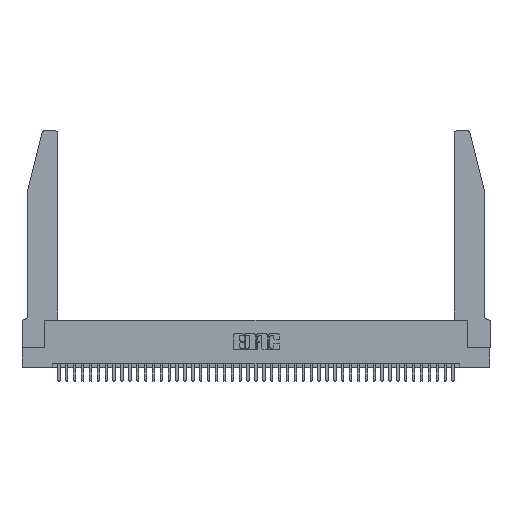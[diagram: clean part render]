
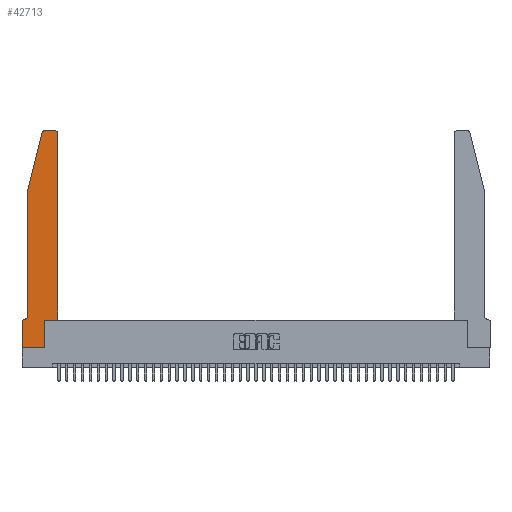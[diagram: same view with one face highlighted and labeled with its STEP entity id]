
A CAD part, top view. The second image highlights one B-rep face of the part: STEP entity #42713.
In plain terms, the highlighted planar face has unit normal (0, 0, 1).
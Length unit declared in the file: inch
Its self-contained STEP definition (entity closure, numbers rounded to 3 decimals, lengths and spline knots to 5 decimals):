
#210 = EDGE_CURVE ( 'NONE', #33803, #3061, #4650, .T. ) ;
#234 = VECTOR ( 'NONE', #22445, 39.37008 ) ;
#853 = DIRECTION ( 'NONE',  ( 1., 0., 0. ) ) ;
#1028 = EDGE_CURVE ( 'NONE', #3170, #3610, #22597, .T. ) ;
#1402 = ORIENTED_EDGE ( 'NONE', *, *, #32171, .T. ) ;
#1412 = VERTEX_POINT ( 'NONE', #35354 ) ;
#1661 = DIRECTION ( 'NONE',  ( 1., 0., 0. ) ) ;
#1755 = ORIENTED_EDGE ( 'NONE', *, *, #35475, .T. ) ;
#2076 = CARTESIAN_POINT ( 'NONE',  ( 0.4505, 0.35, 0.37 ) ) ;
#2695 = LINE ( 'NONE', #10277, #16411 ) ;
#3061 = VERTEX_POINT ( 'NONE', #4089 ) ;
#3170 = VERTEX_POINT ( 'NONE', #8322 ) ;
#3610 = VERTEX_POINT ( 'NONE', #16871 ) ;
#3651 = CARTESIAN_POINT ( 'NONE',  ( 0.284, 2.72, 0.37 ) ) ;
#4089 = CARTESIAN_POINT ( 'NONE',  ( 0.4505, 0.35, 0.37 ) ) ;
#4650 = LINE ( 'NONE', #28960, #7803 ) ;
#5351 = DIRECTION ( 'NONE',  ( -1., 0., 0. ) ) ;
#5510 = DIRECTION ( 'NONE',  ( -0.239, -0.971, 0. ) ) ;
#5765 = VECTOR ( 'NONE', #33285, 39.37008 ) ;
#6436 = DIRECTION ( 'NONE',  ( 0., -1., 0. ) ) ;
#6852 = ORIENTED_EDGE ( 'NONE', *, *, #40280, .T. ) ;
#7072 = AXIS2_PLACEMENT_3D ( 'NONE', #19152, #12638, #22562 ) ;
#7702 = ORIENTED_EDGE ( 'NONE', *, *, #210, .T. ) ;
#7803 = VECTOR ( 'NONE', #1661, 39.37008 ) ;
#8322 = CARTESIAN_POINT ( 'NONE',  ( 0.0755, 2., 0.37 ) ) ;
#8665 = ORIENTED_EDGE ( 'NONE', *, *, #29667, .T. ) ;
#9045 = CARTESIAN_POINT ( 'NONE',  ( 0.2865, 0.35, 0.37 ) ) ;
#9148 = DIRECTION ( 'NONE',  ( 0., 0., 1. ) ) ;
#9233 = CIRCLE ( 'NONE', #14042, 0.03 ) ;
#10057 = ORIENTED_EDGE ( 'NONE', *, *, #18216, .T. ) ;
#10277 = CARTESIAN_POINT ( 'NONE',  ( 0., 0., 0.37 ) ) ;
#11671 = CARTESIAN_POINT ( 'NONE',  ( 0.0755, 2., 0.37 ) ) ;
#12036 = EDGE_CURVE ( 'NONE', #3610, #27990, #17361, .T. ) ;
#12462 = VECTOR ( 'NONE', #39123, 39.37008 ) ;
#12638 = DIRECTION ( 'NONE',  ( 0., 0., 1. ) ) ;
#13542 = EDGE_CURVE ( 'NONE', #27990, #29361, #26884, .T. ) ;
#13628 = CARTESIAN_POINT ( 'NONE',  ( 0., 0.35, 0.37 ) ) ;
#13631 = CARTESIAN_POINT ( 'NONE',  ( 0.2605, 2.75, 0.37 ) ) ;
#14042 = AXIS2_PLACEMENT_3D ( 'NONE', #3651, #20443, #853 ) ;
#14586 = LINE ( 'NONE', #27239, #39975 ) ;
#16258 = AXIS2_PLACEMENT_3D ( 'NONE', #22179, #18629, #5351 ) ;
#16411 = VECTOR ( 'NONE', #20325, 39.37008 ) ;
#16871 = CARTESIAN_POINT ( 'NONE',  ( 0.0755, 0.42, 0.37 ) ) ;
#16915 = LINE ( 'NONE', #13631, #31182 ) ;
#17361 = CIRCLE ( 'NONE', #16258, 0.07 ) ;
#18216 = EDGE_CURVE ( 'NONE', #20698, #27468, #35424, .T. ) ;
#18585 = VERTEX_POINT ( 'NONE', #20320 ) ;
#18629 = DIRECTION ( 'NONE',  ( 0., 0., -1. ) ) ;
#19026 = CARTESIAN_POINT ( 'NONE',  ( 0., 0., 0.37 ) ) ;
#19152 = CARTESIAN_POINT ( 'NONE',  ( 0.4205, 2.72, 0.37 ) ) ;
#20320 = CARTESIAN_POINT ( 'NONE',  ( 0.284, 2.75, 0.37 ) ) ;
#20325 = DIRECTION ( 'NONE',  ( 1., 0., 0. ) ) ;
#20443 = DIRECTION ( 'NONE',  ( 0., 0., 1. ) ) ;
#20698 = VERTEX_POINT ( 'NONE', #42739 ) ;
#21460 = ORIENTED_EDGE ( 'NONE', *, *, #31277, .T. ) ;
#21633 = VERTEX_POINT ( 'NONE', #28605 ) ;
#22179 = CARTESIAN_POINT ( 'NONE',  ( 0.0055, 0.42, 0.37 ) ) ;
#22445 = DIRECTION ( 'NONE',  ( 0., -1., 0. ) ) ;
#22562 = DIRECTION ( 'NONE',  ( 1., 0., 0. ) ) ;
#22597 = LINE ( 'NONE', #39824, #29956 ) ;
#22601 = DIRECTION ( 'NONE',  ( 1., 0., 0. ) ) ;
#22901 = LINE ( 'NONE', #19026, #234 ) ;
#23002 = EDGE_CURVE ( 'NONE', #29361, #21633, #22901, .T. ) ;
#23871 = ORIENTED_EDGE ( 'NONE', *, *, #25536, .T. ) ;
#25536 = EDGE_CURVE ( 'NONE', #18585, #27780, #9233, .T. ) ;
#26274 = CARTESIAN_POINT ( 'NONE',  ( 0., 0.35, 0.37 ) ) ;
#26476 = ORIENTED_EDGE ( 'NONE', *, *, #23002, .T. ) ;
#26651 = DIRECTION ( 'NONE',  ( -1., 0., 0. ) ) ;
#26884 = LINE ( 'NONE', #40075, #5765 ) ;
#27239 = CARTESIAN_POINT ( 'NONE',  ( 0.2865, 0.35, 0.37 ) ) ;
#27468 = VERTEX_POINT ( 'NONE', #33728 ) ;
#27780 = VERTEX_POINT ( 'NONE', #42578 ) ;
#27965 = LINE ( 'NONE', #11671, #37992 ) ;
#27990 = VERTEX_POINT ( 'NONE', #40789 ) ;
#28605 = CARTESIAN_POINT ( 'NONE',  ( 0., 0., 0.37 ) ) ;
#28960 = CARTESIAN_POINT ( 'NONE',  ( 0.4505, 0.35, 0.37 ) ) ;
#28975 = ORIENTED_EDGE ( 'NONE', *, *, #13542, .T. ) ;
#29361 = VERTEX_POINT ( 'NONE', #13628 ) ;
#29667 = EDGE_CURVE ( 'NONE', #27780, #3170, #27965, .T. ) ;
#29668 = AXIS2_PLACEMENT_3D ( 'NONE', #26274, #9148, #22601 ) ;
#29956 = VECTOR ( 'NONE', #6436, 39.37008 ) ;
#31182 = VECTOR ( 'NONE', #26651, 39.37008 ) ;
#31277 = EDGE_CURVE ( 'NONE', #3061, #20698, #39443, .T. ) ;
#32171 = EDGE_CURVE ( 'NONE', #27468, #18585, #16915, .T. ) ;
#33285 = DIRECTION ( 'NONE',  ( -1., 0., 0. ) ) ;
#33728 = CARTESIAN_POINT ( 'NONE',  ( 0.4205, 2.75, 0.37 ) ) ;
#33803 = VERTEX_POINT ( 'NONE', #9045 ) ;
#35354 = CARTESIAN_POINT ( 'NONE',  ( 0.2865, 0., 0.37 ) ) ;
#35424 = CIRCLE ( 'NONE', #7072, 0.03 ) ;
#35475 = EDGE_CURVE ( 'NONE', #1412, #33803, #14586, .T. ) ;
#37437 = DIRECTION ( 'NONE',  ( 0., 1., 0. ) ) ;
#37864 = FACE_OUTER_BOUND ( 'NONE', #41578, .T. ) ;
#37992 = VECTOR ( 'NONE', #5510, 39.37008 ) ;
#39123 = DIRECTION ( 'NONE',  ( 0., 1., 0. ) ) ;
#39443 = LINE ( 'NONE', #2076, #12462 ) ;
#39824 = CARTESIAN_POINT ( 'NONE',  ( 0.0755, 2., 0.37 ) ) ;
#39975 = VECTOR ( 'NONE', #37437, 39.37008 ) ;
#40021 = PLANE ( 'NONE',  #29668 ) ;
#40075 = CARTESIAN_POINT ( 'NONE',  ( 0.0755, 0.35, 0.37 ) ) ;
#40280 = EDGE_CURVE ( 'NONE', #21633, #1412, #2695, .T. ) ;
#40789 = CARTESIAN_POINT ( 'NONE',  ( 0.0055, 0.35, 0.37 ) ) ;
#41578 = EDGE_LOOP ( 'NONE', ( #1402, #23871, #8665, #42365, #42413, #28975, #26476, #6852, #1755, #7702, #21460, #10057 ) ) ;
#42365 = ORIENTED_EDGE ( 'NONE', *, *, #1028, .T. ) ;
#42413 = ORIENTED_EDGE ( 'NONE', *, *, #12036, .T. ) ;
#42578 = CARTESIAN_POINT ( 'NONE',  ( 0.25487, 2.72718, 0.37 ) ) ;
#42713 = ADVANCED_FACE ( 'NONE', ( #37864 ), #40021, .T. ) ;
#42739 = CARTESIAN_POINT ( 'NONE',  ( 0.4505, 2.72, 0.37 ) ) ;
